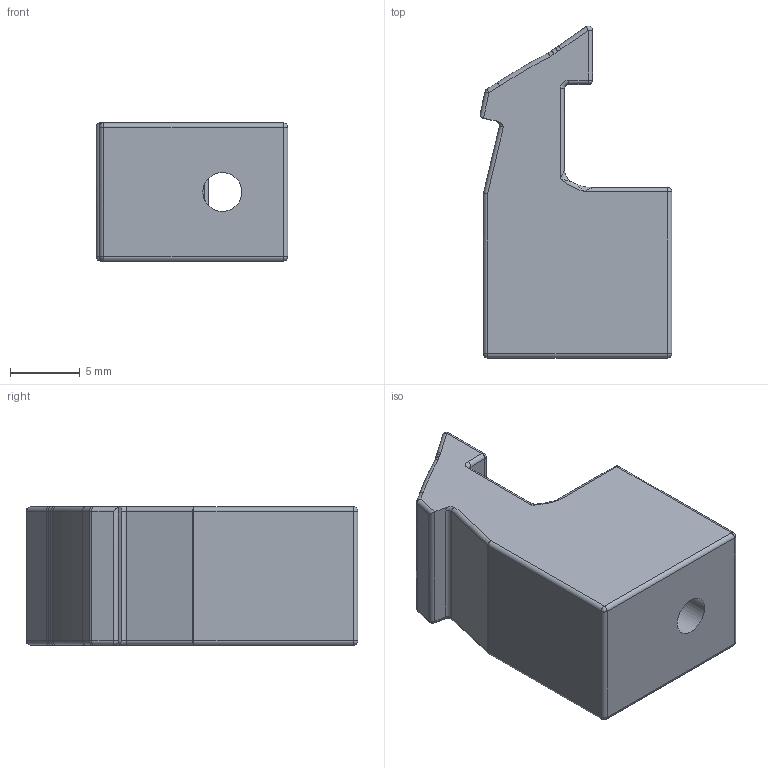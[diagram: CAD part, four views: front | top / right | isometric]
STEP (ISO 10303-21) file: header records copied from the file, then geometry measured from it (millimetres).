
FILE_DESCRIPTION(/* description */ (''),/* implementation_level */ '2;1');
FILE_NAME(/* name */ 'Feed Ramp.step',/* time_stamp */ '2022-05-12T09:37:46-06:00',/* author */ (''),/* organization */ (''),/* preprocessor_version */ 'ST-DEVELOPER v18.1',/* originating_system */ 'Autodesk Translation Framework v10.10.0.1391',/* authorisation */ '');
FILE_SCHEMA (('AUTOMOTIVE_DESIGN { 1 0 10303 214 3 1 1 }'));
Length unit declared in the file: millimetre
Products named in the file (1): Feed Ramp
Bounding box: 13.73 x 23.78 x 9.9 mm (x, y, z)
Volume: 2099.4 mm3; surface area: 1256.9 mm2
Topology: 1 solids, 1 shells, 88 faces, 190 edges, 99 vertices
Faces by surface type: cylinder 41, sphere 15, plane 14, torus 13, bspline 5
Full cylindrical faces by diameter (mm): 2.8 x1
Entity records: 2549 total; most frequent: CARTESIAN_POINT 609, DIRECTION 440, ORIENTED_EDGE 372, EDGE_CURVE 186, AXIS2_PLACEMENT_3D 181, VERTEX_POINT 99, CIRCLE 94, EDGE_LOOP 89
